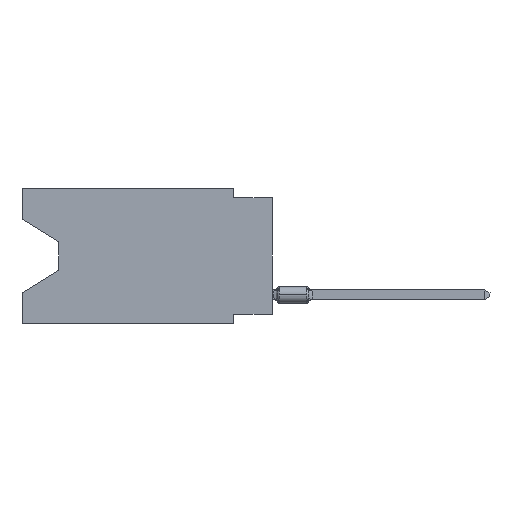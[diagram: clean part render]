
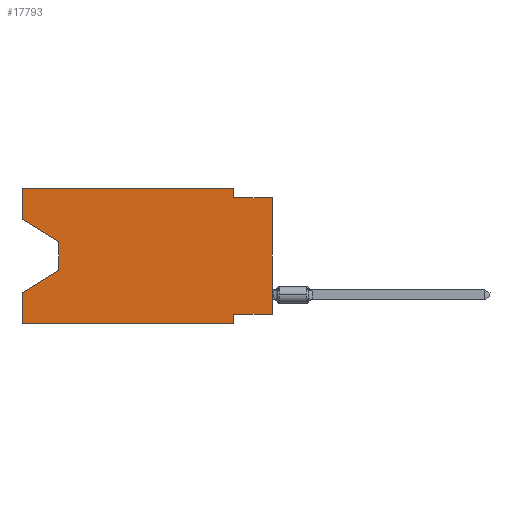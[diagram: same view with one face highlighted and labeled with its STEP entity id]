
A CAD part, left-side view. The second image highlights one B-rep face of the part: STEP entity #17793.
In plain terms, the highlighted planar face has unit normal (-1, 0, 0).
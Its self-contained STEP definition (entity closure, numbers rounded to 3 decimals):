
#361 = ORIENTED_EDGE ( 'NONE', *, *, #3139, .F. ) ;
#566 = LINE ( 'NONE', #11458, #15796 ) ;
#1071 = VERTEX_POINT ( 'NONE', #25768 ) ;
#1301 = DIRECTION ( 'NONE',  ( 0., 0., 1. ) ) ;
#1485 = VECTOR ( 'NONE', #20732, 1000. ) ;
#1666 = EDGE_CURVE ( 'NONE', #22772, #5143, #22459, .T. ) ;
#1771 = VECTOR ( 'NONE', #5936, 1000. ) ;
#2035 = CARTESIAN_POINT ( 'NONE',  ( 0., 0., -0.635 ) ) ;
#2289 = VERTEX_POINT ( 'NONE', #18133 ) ;
#2982 = ORIENTED_EDGE ( 'NONE', *, *, #14702, .T. ) ;
#3126 = LINE ( 'NONE', #11854, #11313 ) ;
#3139 = EDGE_CURVE ( 'NONE', #20984, #11466, #8223, .T. ) ;
#3368 = DIRECTION ( 'NONE',  ( 0., 0., 1. ) ) ;
#3651 = ORIENTED_EDGE ( 'NONE', *, *, #14980, .F. ) ;
#3766 = CARTESIAN_POINT ( 'NONE',  ( 0., 13.97, -3.505 ) ) ;
#3895 = ORIENTED_EDGE ( 'NONE', *, *, #10312, .F. ) ;
#4066 = VERTEX_POINT ( 'NONE', #25422 ) ;
#4133 = VECTOR ( 'NONE', #3368, 1000. ) ;
#5092 = CARTESIAN_POINT ( 'NONE',  ( 0., 2.54, -0.635 ) ) ;
#5143 = VERTEX_POINT ( 'NONE', #10261 ) ;
#5386 = EDGE_CURVE ( 'NONE', #1071, #22772, #3126, .T. ) ;
#5524 = CARTESIAN_POINT ( 'NONE',  ( 0., 2.54, -8.255 ) ) ;
#5547 = DIRECTION ( 'NONE',  ( 0., 0., -1. ) ) ;
#5913 = CARTESIAN_POINT ( 'NONE',  ( 0., 0., -0.635 ) ) ;
#5936 = DIRECTION ( 'NONE',  ( 0., 0., -1. ) ) ;
#6181 = VECTOR ( 'NONE', #5547, 1000. ) ;
#6215 = VECTOR ( 'NONE', #7283, 1000. ) ;
#6776 = EDGE_CURVE ( 'NONE', #4066, #13402, #8133, .T. ) ;
#6913 = ORIENTED_EDGE ( 'NONE', *, *, #5386, .T. ) ;
#7213 = LINE ( 'NONE', #23737, #13660 ) ;
#7283 = DIRECTION ( 'NONE',  ( 0., 0., 1. ) ) ;
#7734 = PLANE ( 'NONE',  #25562 ) ;
#8106 = LINE ( 'NONE', #5913, #21147 ) ;
#8133 = LINE ( 'NONE', #24771, #18009 ) ;
#8223 = LINE ( 'NONE', #20373, #16924 ) ;
#8307 = CARTESIAN_POINT ( 'NONE',  ( 0., 2.54, -8.89 ) ) ;
#8991 = LINE ( 'NONE', #18113, #22797 ) ;
#9675 = DIRECTION ( 'NONE',  ( 0., -0.855, -0.519 ) ) ;
#10261 = CARTESIAN_POINT ( 'NONE',  ( 0., 13.97, -5.385 ) ) ;
#10312 = EDGE_CURVE ( 'NONE', #21671, #18863, #14018, .T. ) ;
#11313 = VECTOR ( 'NONE', #9675, 1000. ) ;
#11458 = CARTESIAN_POINT ( 'NONE',  ( 0., 16.383, 0. ) ) ;
#11466 = VERTEX_POINT ( 'NONE', #5524 ) ;
#11558 = DIRECTION ( 'NONE',  ( 0., 0., -1. ) ) ;
#11854 = CARTESIAN_POINT ( 'NONE',  ( 0., 16.383, -2.038 ) ) ;
#11924 = DIRECTION ( 'NONE',  ( 0., -1., 0. ) ) ;
#12489 = EDGE_CURVE ( 'NONE', #24196, #21671, #566, .T. ) ;
#12561 = ORIENTED_EDGE ( 'NONE', *, *, #26991, .T. ) ;
#13104 = CARTESIAN_POINT ( 'NONE',  ( 0., 16.383, 0. ) ) ;
#13402 = VERTEX_POINT ( 'NONE', #24513 ) ;
#13660 = VECTOR ( 'NONE', #17193, 1000. ) ;
#14018 = LINE ( 'NONE', #22333, #6181 ) ;
#14022 = FACE_OUTER_BOUND ( 'NONE', #14569, .T. ) ;
#14341 = ORIENTED_EDGE ( 'NONE', *, *, #22549, .F. ) ;
#14569 = EDGE_LOOP ( 'NONE', ( #6913, #23454, #2982, #20305, #12561, #3651, #361, #22205, #14341, #3895, #20179, #24612 ) ) ;
#14702 = EDGE_CURVE ( 'NONE', #5143, #13402, #7213, .T. ) ;
#14980 = EDGE_CURVE ( 'NONE', #11466, #2289, #22626, .T. ) ;
#15562 = DIRECTION ( 'NONE',  ( 0., -1., 0. ) ) ;
#15796 = VECTOR ( 'NONE', #15562, 1000. ) ;
#16924 = VECTOR ( 'NONE', #24858, 1000. ) ;
#17193 = DIRECTION ( 'NONE',  ( 0., 0.855, -0.519 ) ) ;
#17793 = ADVANCED_FACE ( 'NONE', ( #14022 ), #7734, .F. ) ;
#17833 = CARTESIAN_POINT ( 'NONE',  ( 0., 16.383, 0. ) ) ;
#18009 = VECTOR ( 'NONE', #1301, 1000. ) ;
#18113 = CARTESIAN_POINT ( 'NONE',  ( 0., 16.383, -8.89 ) ) ;
#18133 = CARTESIAN_POINT ( 'NONE',  ( 0., 2.54, -8.89 ) ) ;
#18863 = VERTEX_POINT ( 'NONE', #5092 ) ;
#19031 = CARTESIAN_POINT ( 'NONE',  ( 0., 13.97, -3.505 ) ) ;
#20147 = LINE ( 'NONE', #13104, #4133 ) ;
#20179 = ORIENTED_EDGE ( 'NONE', *, *, #12489, .F. ) ;
#20305 = ORIENTED_EDGE ( 'NONE', *, *, #6776, .F. ) ;
#20373 = CARTESIAN_POINT ( 'NONE',  ( 0., 0., -8.255 ) ) ;
#20732 = DIRECTION ( 'NONE',  ( 0., 0., -1. ) ) ;
#20984 = VERTEX_POINT ( 'NONE', #25534 ) ;
#21147 = VECTOR ( 'NONE', #11924, 1000. ) ;
#21671 = VERTEX_POINT ( 'NONE', #26021 ) ;
#22014 = EDGE_CURVE ( 'NONE', #1071, #24196, #20147, .T. ) ;
#22205 = ORIENTED_EDGE ( 'NONE', *, *, #26325, .T. ) ;
#22333 = CARTESIAN_POINT ( 'NONE',  ( 0., 2.54, 0. ) ) ;
#22459 = LINE ( 'NONE', #3766, #1771 ) ;
#22549 = EDGE_CURVE ( 'NONE', #18863, #25553, #8106, .T. ) ;
#22626 = LINE ( 'NONE', #8307, #1485 ) ;
#22772 = VERTEX_POINT ( 'NONE', #19031 ) ;
#22797 = VECTOR ( 'NONE', #25882, 1000. ) ;
#23454 = ORIENTED_EDGE ( 'NONE', *, *, #1666, .T. ) ;
#23737 = CARTESIAN_POINT ( 'NONE',  ( 0., 13.97, -5.385 ) ) ;
#24130 = CARTESIAN_POINT ( 'NONE',  ( 0., 16.383, 0. ) ) ;
#24196 = VERTEX_POINT ( 'NONE', #24130 ) ;
#24378 = DIRECTION ( 'NONE',  ( 1., 0., 0. ) ) ;
#24513 = CARTESIAN_POINT ( 'NONE',  ( 0., 16.383, -6.852 ) ) ;
#24612 = ORIENTED_EDGE ( 'NONE', *, *, #22014, .F. ) ;
#24771 = CARTESIAN_POINT ( 'NONE',  ( 0., 16.383, 0. ) ) ;
#24858 = DIRECTION ( 'NONE',  ( 0., 1., 0. ) ) ;
#25422 = CARTESIAN_POINT ( 'NONE',  ( 0., 16.383, -8.89 ) ) ;
#25534 = CARTESIAN_POINT ( 'NONE',  ( 0., 0., -8.255 ) ) ;
#25553 = VERTEX_POINT ( 'NONE', #2035 ) ;
#25562 = AXIS2_PLACEMENT_3D ( 'NONE', #17833, #24378, #11558 ) ;
#25768 = CARTESIAN_POINT ( 'NONE',  ( 0., 16.383, -2.038 ) ) ;
#25882 = DIRECTION ( 'NONE',  ( 0., -1., 0. ) ) ;
#25971 = LINE ( 'NONE', #26104, #6215 ) ;
#26021 = CARTESIAN_POINT ( 'NONE',  ( 0., 2.54, 0. ) ) ;
#26104 = CARTESIAN_POINT ( 'NONE',  ( 0., 0., 0. ) ) ;
#26325 = EDGE_CURVE ( 'NONE', #20984, #25553, #25971, .T. ) ;
#26991 = EDGE_CURVE ( 'NONE', #4066, #2289, #8991, .T. ) ;
